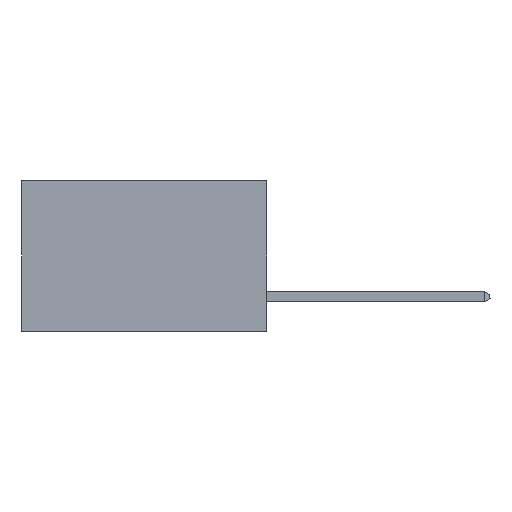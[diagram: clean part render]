
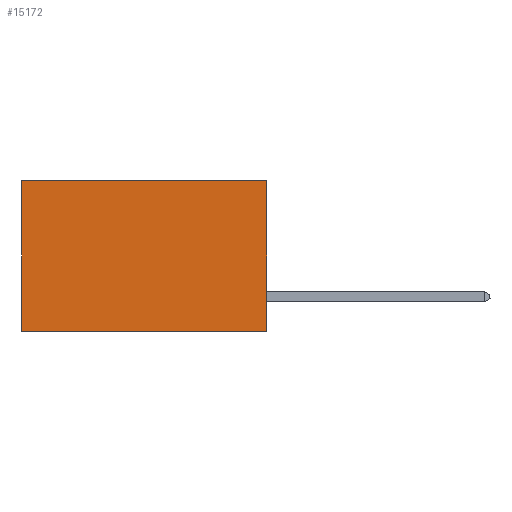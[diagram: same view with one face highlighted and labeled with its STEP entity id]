
A CAD part, left-side view. The second image highlights one B-rep face of the part: STEP entity #15172.
In plain terms, the highlighted planar face has unit normal (-1, 0, 0).
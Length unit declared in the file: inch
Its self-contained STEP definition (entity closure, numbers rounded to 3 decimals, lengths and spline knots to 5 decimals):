
#1962 = ORIENTED_EDGE ( 'NONE', *, *, #3177, .T. ) ;
#2314 = CARTESIAN_POINT ( 'NONE',  ( 0.2875, 0., -0.37 ) ) ;
#3177 = EDGE_CURVE ( 'NONE', #16751, #6379, #11855, .T. ) ;
#3824 = ORIENTED_EDGE ( 'NONE', *, *, #13560, .T. ) ;
#4816 = LINE ( 'NONE', #7324, #16840 ) ;
#5029 = CARTESIAN_POINT ( 'NONE',  ( 0.2875, 0., 0. ) ) ;
#5105 = ORIENTED_EDGE ( 'NONE', *, *, #19314, .F. ) ;
#5392 = VECTOR ( 'NONE', #20119, 39.37008 ) ;
#5807 = VECTOR ( 'NONE', #18656, 39.37008 ) ;
#5949 = DIRECTION ( 'NONE',  ( 1., 0., 0. ) ) ;
#6379 = VERTEX_POINT ( 'NONE', #13742 ) ;
#7293 = VECTOR ( 'NONE', #20899, 39.37008 ) ;
#7324 = CARTESIAN_POINT ( 'NONE',  ( 0.2875, 0., 0. ) ) ;
#8500 = VERTEX_POINT ( 'NONE', #20846 ) ;
#9083 = DIRECTION ( 'NONE',  ( 0., 0., -1. ) ) ;
#9479 = EDGE_LOOP ( 'NONE', ( #3824, #18394, #5105, #1962 ) ) ;
#9838 = FACE_OUTER_BOUND ( 'NONE', #9479, .T. ) ;
#10311 = EDGE_CURVE ( 'NONE', #14469, #8500, #19316, .T. ) ;
#11855 = LINE ( 'NONE', #20828, #7293 ) ;
#12127 = AXIS2_PLACEMENT_3D ( 'NONE', #21097, #5949, #17856 ) ;
#13560 = EDGE_CURVE ( 'NONE', #6379, #8500, #14505, .T. ) ;
#13742 = CARTESIAN_POINT ( 'NONE',  ( 0.2875, 0.6, 0. ) ) ;
#14469 = VERTEX_POINT ( 'NONE', #2314 ) ;
#14505 = LINE ( 'NONE', #18459, #5392 ) ;
#15172 = ADVANCED_FACE ( 'NONE', ( #9838 ), #16199, .F. ) ;
#16199 = PLANE ( 'NONE',  #12127 ) ;
#16751 = VERTEX_POINT ( 'NONE', #5029 ) ;
#16840 = VECTOR ( 'NONE', #9083, 39.37008 ) ;
#17856 = DIRECTION ( 'NONE',  ( 0., 0., -1. ) ) ;
#18394 = ORIENTED_EDGE ( 'NONE', *, *, #10311, .F. ) ;
#18459 = CARTESIAN_POINT ( 'NONE',  ( 0.2875, 0.6, 0. ) ) ;
#18656 = DIRECTION ( 'NONE',  ( 0., 1., 0. ) ) ;
#19314 = EDGE_CURVE ( 'NONE', #16751, #14469, #4816, .T. ) ;
#19316 = LINE ( 'NONE', #20399, #5807 ) ;
#20119 = DIRECTION ( 'NONE',  ( 0., 0., -1. ) ) ;
#20399 = CARTESIAN_POINT ( 'NONE',  ( 0.2875, 0., -0.37 ) ) ;
#20828 = CARTESIAN_POINT ( 'NONE',  ( 0.2875, 0., 0. ) ) ;
#20846 = CARTESIAN_POINT ( 'NONE',  ( 0.2875, 0.6, -0.37 ) ) ;
#20899 = DIRECTION ( 'NONE',  ( 0., 1., 0. ) ) ;
#21097 = CARTESIAN_POINT ( 'NONE',  ( 0.2875, 0., 0. ) ) ;
